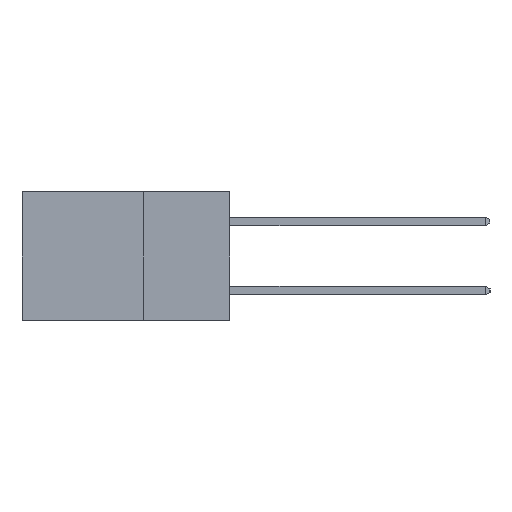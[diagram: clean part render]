
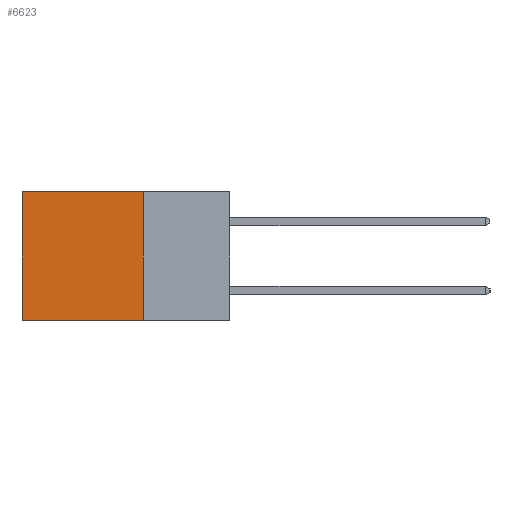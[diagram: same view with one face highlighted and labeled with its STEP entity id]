
A CAD part, left-side view. The second image highlights one B-rep face of the part: STEP entity #6623.
In plain terms, the highlighted planar face has unit normal (-1, 0, 0).
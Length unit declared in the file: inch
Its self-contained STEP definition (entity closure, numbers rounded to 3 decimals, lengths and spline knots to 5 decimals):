
#566 = ORIENTED_EDGE ( 'NONE', *, *, #7014, .T. ) ;
#881 = VERTEX_POINT ( 'NONE', #7694 ) ;
#910 = ORIENTED_EDGE ( 'NONE', *, *, #9642, .T. ) ;
#1082 = VECTOR ( 'NONE', #10009, 39.37008 ) ;
#1657 = DIRECTION ( 'NONE',  ( 0., 0., -1. ) ) ;
#1671 = DIRECTION ( 'NONE',  ( 1., 0., 0. ) ) ;
#1690 = CARTESIAN_POINT ( 'NONE',  ( 0.2615, 0.25, -0.37 ) ) ;
#1878 = PLANE ( 'NONE',  #5286 ) ;
#2156 = VERTEX_POINT ( 'NONE', #2795 ) ;
#2360 = DIRECTION ( 'NONE',  ( 0., 0., -1. ) ) ;
#2451 = CARTESIAN_POINT ( 'NONE',  ( 0.2615, 0.25, -0.37 ) ) ;
#2795 = CARTESIAN_POINT ( 'NONE',  ( 0.2615, 0.6, -0.37 ) ) ;
#2940 = LINE ( 'NONE', #3599, #8250 ) ;
#2949 = VECTOR ( 'NONE', #2360, 39.37008 ) ;
#3408 = DIRECTION ( 'NONE',  ( 0., 1., 0. ) ) ;
#3547 = ORIENTED_EDGE ( 'NONE', *, *, #5398, .F. ) ;
#3599 = CARTESIAN_POINT ( 'NONE',  ( 0.2615, 0.25, 0. ) ) ;
#4273 = VECTOR ( 'NONE', #5421, 39.37008 ) ;
#4534 = CARTESIAN_POINT ( 'NONE',  ( 0.2615, 0.6, 0. ) ) ;
#5217 = VERTEX_POINT ( 'NONE', #4534 ) ;
#5286 = AXIS2_PLACEMENT_3D ( 'NONE', #1690, #1671, #1657 ) ;
#5398 = EDGE_CURVE ( 'NONE', #881, #2156, #13016, .T. ) ;
#5421 = DIRECTION ( 'NONE',  ( 0., 1., 0. ) ) ;
#6102 = EDGE_LOOP ( 'NONE', ( #566, #3547, #12312, #910 ) ) ;
#6623 = ADVANCED_FACE ( 'NONE', ( #8937 ), #1878, .F. ) ;
#6990 = CARTESIAN_POINT ( 'NONE',  ( 0.2615, 0.25, -0.37 ) ) ;
#7014 = EDGE_CURVE ( 'NONE', #5217, #2156, #12802, .T. ) ;
#7681 = CARTESIAN_POINT ( 'NONE',  ( 0.2615, 0.25, 0. ) ) ;
#7694 = CARTESIAN_POINT ( 'NONE',  ( 0.2615, 0.25, -0.37 ) ) ;
#8250 = VECTOR ( 'NONE', #3408, 39.37008 ) ;
#8937 = FACE_OUTER_BOUND ( 'NONE', #6102, .T. ) ;
#9337 = CARTESIAN_POINT ( 'NONE',  ( 0.2615, 0.6, -0.37 ) ) ;
#9642 = EDGE_CURVE ( 'NONE', #10861, #5217, #2940, .T. ) ;
#10009 = DIRECTION ( 'NONE',  ( 0., 0., -1. ) ) ;
#10861 = VERTEX_POINT ( 'NONE', #7681 ) ;
#11391 = LINE ( 'NONE', #2451, #2949 ) ;
#11658 = EDGE_CURVE ( 'NONE', #10861, #881, #11391, .T. ) ;
#12312 = ORIENTED_EDGE ( 'NONE', *, *, #11658, .F. ) ;
#12802 = LINE ( 'NONE', #9337, #1082 ) ;
#13016 = LINE ( 'NONE', #6990, #4273 ) ;
